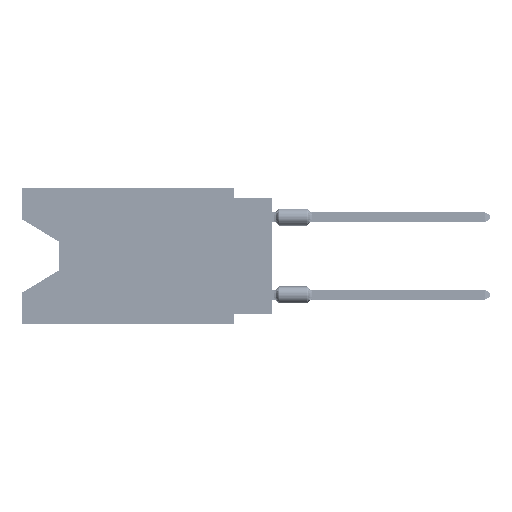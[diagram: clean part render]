
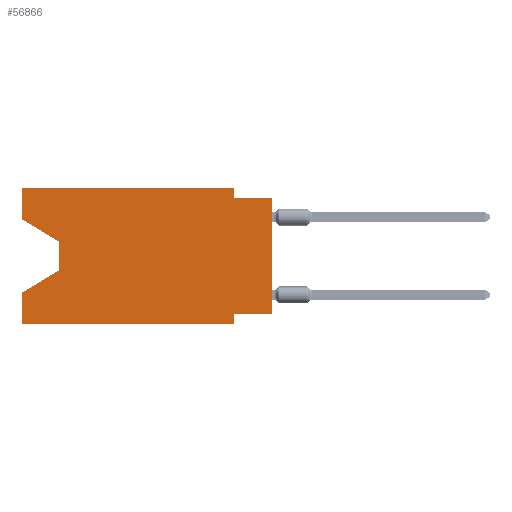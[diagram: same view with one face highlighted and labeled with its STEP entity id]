
A CAD part, left-side view. The second image highlights one B-rep face of the part: STEP entity #56866.
In plain terms, the highlighted planar face has unit normal (-1, 0, 0).
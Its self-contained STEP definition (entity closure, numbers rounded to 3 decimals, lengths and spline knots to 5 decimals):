
#168 = DIRECTION ( 'NONE',  ( 0., -0.855, -0.519 ) ) ;
#756 = CARTESIAN_POINT ( 'NONE',  ( 0., 0.645, -0.08025 ) ) ;
#1413 = DIRECTION ( 'NONE',  ( 0., -1., 0. ) ) ;
#4257 = ORIENTED_EDGE ( 'NONE', *, *, #32163, .F. ) ;
#7681 = VERTEX_POINT ( 'NONE', #15803 ) ;
#8509 = EDGE_CURVE ( 'NONE', #94667, #7681, #18314, .T. ) ;
#12796 = DIRECTION ( 'NONE',  ( 0., 0., -1. ) ) ;
#14976 = ORIENTED_EDGE ( 'NONE', *, *, #77606, .T. ) ;
#15772 = ORIENTED_EDGE ( 'NONE', *, *, #79648, .F. ) ;
#15803 = CARTESIAN_POINT ( 'NONE',  ( 0., 0.55, -0.138 ) ) ;
#16464 = CARTESIAN_POINT ( 'NONE',  ( 0., 0.645, 0. ) ) ;
#17619 = EDGE_CURVE ( 'NONE', #104771, #75550, #95802, .T. ) ;
#18314 = LINE ( 'NONE', #756, #98161 ) ;
#18474 = DIRECTION ( 'NONE',  ( 0., 1., 0. ) ) ;
#18865 = CARTESIAN_POINT ( 'NONE',  ( 0., 0.645, 0. ) ) ;
#20621 = VECTOR ( 'NONE', #79008, 39.37008 ) ;
#25345 = VECTOR ( 'NONE', #86519, 39.37008 ) ;
#25696 = LINE ( 'NONE', #104649, #25345 ) ;
#27851 = EDGE_CURVE ( 'NONE', #87054, #75550, #92997, .T. ) ;
#30359 = ORIENTED_EDGE ( 'NONE', *, *, #69992, .F. ) ;
#31922 = LINE ( 'NONE', #103295, #74739 ) ;
#32163 = EDGE_CURVE ( 'NONE', #94667, #61314, #82578, .T. ) ;
#32242 = ORIENTED_EDGE ( 'NONE', *, *, #103190, .F. ) ;
#33384 = CARTESIAN_POINT ( 'NONE',  ( 0., 0.645, -0.26975 ) ) ;
#33626 = DIRECTION ( 'NONE',  ( 0., 0., 1. ) ) ;
#33767 = VERTEX_POINT ( 'NONE', #33384 ) ;
#33994 = VECTOR ( 'NONE', #36982, 39.37008 ) ;
#34772 = LINE ( 'NONE', #80964, #104203 ) ;
#36982 = DIRECTION ( 'NONE',  ( 0., 0., 1. ) ) ;
#39888 = VECTOR ( 'NONE', #78805, 39.37008 ) ;
#43136 = ORIENTED_EDGE ( 'NONE', *, *, #65573, .F. ) ;
#45281 = CARTESIAN_POINT ( 'NONE',  ( 0., 0., -0.025 ) ) ;
#45782 = PLANE ( 'NONE',  #87882 ) ;
#46372 = DIRECTION ( 'NONE',  ( 1., 0., 0. ) ) ;
#46597 = CARTESIAN_POINT ( 'NONE',  ( 0., 0.55, -0.212 ) ) ;
#48590 = ORIENTED_EDGE ( 'NONE', *, *, #17619, .F. ) ;
#48844 = VECTOR ( 'NONE', #64342, 39.37008 ) ;
#48962 = VECTOR ( 'NONE', #98487, 39.37008 ) ;
#52180 = CARTESIAN_POINT ( 'NONE',  ( 0., 0.1, -0.025 ) ) ;
#52683 = LINE ( 'NONE', #16464, #20621 ) ;
#53375 = FACE_OUTER_BOUND ( 'NONE', #92496, .T. ) ;
#55181 = LINE ( 'NONE', #45281, #80825 ) ;
#56866 = ADVANCED_FACE ( 'NONE', ( #53375 ), #45782, .F. ) ;
#57200 = LINE ( 'NONE', #92897, #61540 ) ;
#58808 = CARTESIAN_POINT ( 'NONE',  ( 0., 0.1, -0.325 ) ) ;
#59181 = EDGE_CURVE ( 'NONE', #82122, #33767, #25696, .T. ) ;
#59231 = CARTESIAN_POINT ( 'NONE',  ( 0., 0., -0.025 ) ) ;
#61138 = ORIENTED_EDGE ( 'NONE', *, *, #27851, .T. ) ;
#61314 = VERTEX_POINT ( 'NONE', #96195 ) ;
#61540 = VECTOR ( 'NONE', #12796, 39.37008 ) ;
#62770 = CARTESIAN_POINT ( 'NONE',  ( 0., 0.645, 0. ) ) ;
#62936 = ORIENTED_EDGE ( 'NONE', *, *, #59181, .T. ) ;
#63791 = VECTOR ( 'NONE', #18474, 39.37008 ) ;
#64342 = DIRECTION ( 'NONE',  ( 0., -1., 0. ) ) ;
#65573 = EDGE_CURVE ( 'NONE', #114397, #109894, #57200, .T. ) ;
#65842 = DIRECTION ( 'NONE',  ( 0., 0., -1. ) ) ;
#69992 = EDGE_CURVE ( 'NONE', #77401, #104771, #105599, .T. ) ;
#74436 = CARTESIAN_POINT ( 'NONE',  ( 0., 0.645, -0.35 ) ) ;
#74739 = VECTOR ( 'NONE', #65842, 39.37008 ) ;
#75550 = VERTEX_POINT ( 'NONE', #94182 ) ;
#77401 = VERTEX_POINT ( 'NONE', #77617 ) ;
#77606 = EDGE_CURVE ( 'NONE', #7681, #82122, #31922, .T. ) ;
#77617 = CARTESIAN_POINT ( 'NONE',  ( 0., 0., -0.325 ) ) ;
#78805 = DIRECTION ( 'NONE',  ( 0., 0., -1. ) ) ;
#79008 = DIRECTION ( 'NONE',  ( 0., 0., 1. ) ) ;
#79648 = EDGE_CURVE ( 'NONE', #61314, #114397, #99649, .T. ) ;
#80825 = VECTOR ( 'NONE', #1413, 39.37008 ) ;
#80964 = CARTESIAN_POINT ( 'NONE',  ( 0., 0., 0. ) ) ;
#82122 = VERTEX_POINT ( 'NONE', #46597 ) ;
#82578 = LINE ( 'NONE', #18865, #33994 ) ;
#86519 = DIRECTION ( 'NONE',  ( 0., 0.855, -0.519 ) ) ;
#87010 = CARTESIAN_POINT ( 'NONE',  ( 0., 0.1, -0.35 ) ) ;
#87054 = VERTEX_POINT ( 'NONE', #74436 ) ;
#87882 = AXIS2_PLACEMENT_3D ( 'NONE', #108925, #46372, #89639 ) ;
#89639 = DIRECTION ( 'NONE',  ( 0., 0., -1. ) ) ;
#89854 = EDGE_CURVE ( 'NONE', #77401, #113988, #34772, .T. ) ;
#92496 = EDGE_LOOP ( 'NONE', ( #111109, #14976, #62936, #93196, #61138, #48590, #30359, #109462, #32242, #43136, #15772, #4257 ) ) ;
#92897 = CARTESIAN_POINT ( 'NONE',  ( 0., 0.1, 0. ) ) ;
#92997 = LINE ( 'NONE', #102356, #48844 ) ;
#93196 = ORIENTED_EDGE ( 'NONE', *, *, #94271, .F. ) ;
#94182 = CARTESIAN_POINT ( 'NONE',  ( 0., 0.1, -0.35 ) ) ;
#94271 = EDGE_CURVE ( 'NONE', #87054, #33767, #52683, .T. ) ;
#94667 = VERTEX_POINT ( 'NONE', #103819 ) ;
#95802 = LINE ( 'NONE', #87010, #39888 ) ;
#96195 = CARTESIAN_POINT ( 'NONE',  ( 0., 0.645, 0. ) ) ;
#98161 = VECTOR ( 'NONE', #168, 39.37008 ) ;
#98487 = DIRECTION ( 'NONE',  ( 0., -1., 0. ) ) ;
#98590 = CARTESIAN_POINT ( 'NONE',  ( 0., 0., -0.325 ) ) ;
#99649 = LINE ( 'NONE', #62770, #48962 ) ;
#102356 = CARTESIAN_POINT ( 'NONE',  ( 0., 0.645, -0.35 ) ) ;
#103190 = EDGE_CURVE ( 'NONE', #109894, #113988, #55181, .T. ) ;
#103295 = CARTESIAN_POINT ( 'NONE',  ( 0., 0.55, -0.138 ) ) ;
#103819 = CARTESIAN_POINT ( 'NONE',  ( 0., 0.645, -0.08025 ) ) ;
#104203 = VECTOR ( 'NONE', #33626, 39.37008 ) ;
#104649 = CARTESIAN_POINT ( 'NONE',  ( 0., 0.55, -0.212 ) ) ;
#104771 = VERTEX_POINT ( 'NONE', #58808 ) ;
#105599 = LINE ( 'NONE', #98590, #63791 ) ;
#108925 = CARTESIAN_POINT ( 'NONE',  ( 0., 0.645, 0. ) ) ;
#109462 = ORIENTED_EDGE ( 'NONE', *, *, #89854, .T. ) ;
#109894 = VERTEX_POINT ( 'NONE', #52180 ) ;
#111109 = ORIENTED_EDGE ( 'NONE', *, *, #8509, .T. ) ;
#111167 = CARTESIAN_POINT ( 'NONE',  ( 0., 0.1, 0. ) ) ;
#113988 = VERTEX_POINT ( 'NONE', #59231 ) ;
#114397 = VERTEX_POINT ( 'NONE', #111167 ) ;
